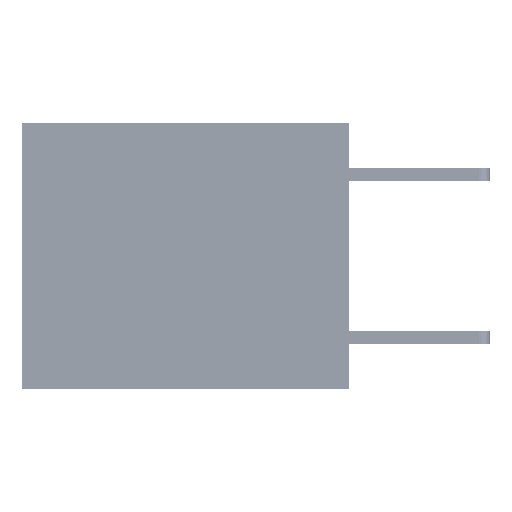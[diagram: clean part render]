
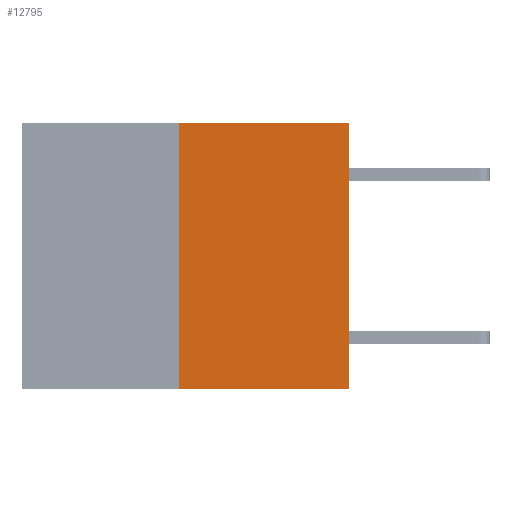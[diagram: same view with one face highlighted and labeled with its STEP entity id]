
A CAD part, left-side view. The second image highlights one B-rep face of the part: STEP entity #12795.
In plain terms, the highlighted planar face has unit normal (-1, 0, 0).
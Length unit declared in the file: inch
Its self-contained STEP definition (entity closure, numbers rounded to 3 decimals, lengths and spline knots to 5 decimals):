
#1140 = LINE ( 'NONE', #31410, #18327 ) ;
#2736 = EDGE_CURVE ( 'NONE', #8884, #13001, #29252, .T. ) ;
#3056 = VECTOR ( 'NONE', #22046, 39.37008 ) ;
#3389 = VECTOR ( 'NONE', #27606, 39.37008 ) ;
#5371 = CARTESIAN_POINT ( 'NONE',  ( 0., 0.312, -0.49 ) ) ;
#6224 = EDGE_CURVE ( 'NONE', #13001, #26440, #32321, .T. ) ;
#6481 = EDGE_CURVE ( 'NONE', #8884, #11084, #1140, .T. ) ;
#7985 = DIRECTION ( 'NONE',  ( 1., 0., 0. ) ) ;
#7995 = ORIENTED_EDGE ( 'NONE', *, *, #6481, .F. ) ;
#8884 = VERTEX_POINT ( 'NONE', #5371 ) ;
#10499 = DIRECTION ( 'NONE',  ( 0., 0., -1. ) ) ;
#11084 = VERTEX_POINT ( 'NONE', #35154 ) ;
#12795 = ADVANCED_FACE ( 'NONE', ( #32319 ), #33124, .F. ) ;
#12985 = LINE ( 'NONE', #22286, #3056 ) ;
#13001 = VERTEX_POINT ( 'NONE', #21351 ) ;
#13004 = CARTESIAN_POINT ( 'NONE',  ( 0., 0.6, -0.49 ) ) ;
#14098 = DIRECTION ( 'NONE',  ( 0., 0., 1. ) ) ;
#15576 = EDGE_LOOP ( 'NONE', ( #7995, #31623, #34778, #16492 ) ) ;
#16492 = ORIENTED_EDGE ( 'NONE', *, *, #31731, .F. ) ;
#18261 = CARTESIAN_POINT ( 'NONE',  ( 0., 0., 0. ) ) ;
#18327 = VECTOR ( 'NONE', #14098, 39.37008 ) ;
#18754 = CARTESIAN_POINT ( 'NONE',  ( 0., 0.6, 0. ) ) ;
#21351 = CARTESIAN_POINT ( 'NONE',  ( 0., 0., -0.49 ) ) ;
#21581 = VECTOR ( 'NONE', #36135, 39.37008 ) ;
#22046 = DIRECTION ( 'NONE',  ( 0., -1., 0. ) ) ;
#22286 = CARTESIAN_POINT ( 'NONE',  ( 0., 0.6, 0. ) ) ;
#26440 = VERTEX_POINT ( 'NONE', #18261 ) ;
#26912 = AXIS2_PLACEMENT_3D ( 'NONE', #18754, #7985, #10499 ) ;
#27606 = DIRECTION ( 'NONE',  ( 0., 0., 1. ) ) ;
#29252 = LINE ( 'NONE', #13004, #21581 ) ;
#31410 = CARTESIAN_POINT ( 'NONE',  ( 0., 0.312, -0.49 ) ) ;
#31623 = ORIENTED_EDGE ( 'NONE', *, *, #2736, .T. ) ;
#31731 = EDGE_CURVE ( 'NONE', #11084, #26440, #12985, .T. ) ;
#32319 = FACE_OUTER_BOUND ( 'NONE', #15576, .T. ) ;
#32321 = LINE ( 'NONE', #32540, #3389 ) ;
#32540 = CARTESIAN_POINT ( 'NONE',  ( 0., 0., 0. ) ) ;
#33124 = PLANE ( 'NONE',  #26912 ) ;
#34778 = ORIENTED_EDGE ( 'NONE', *, *, #6224, .T. ) ;
#35154 = CARTESIAN_POINT ( 'NONE',  ( 0., 0.312, 0. ) ) ;
#36135 = DIRECTION ( 'NONE',  ( 0., -1., 0. ) ) ;
